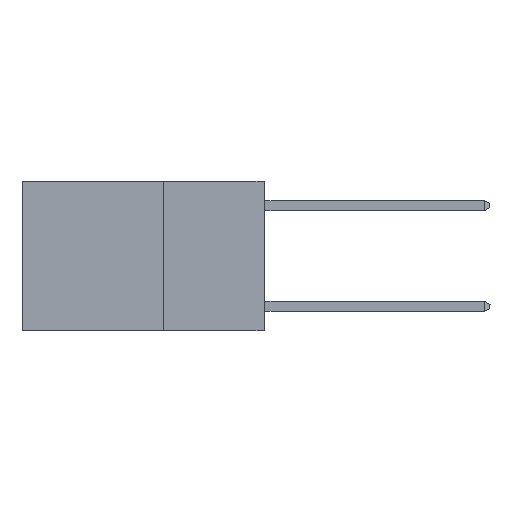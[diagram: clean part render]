
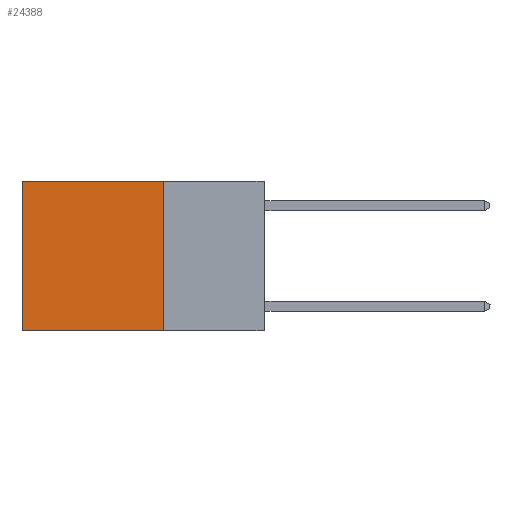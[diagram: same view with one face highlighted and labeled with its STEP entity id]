
A CAD part, left-side view. The second image highlights one B-rep face of the part: STEP entity #24388.
In plain terms, the highlighted planar face has unit normal (-1, 0, 0).
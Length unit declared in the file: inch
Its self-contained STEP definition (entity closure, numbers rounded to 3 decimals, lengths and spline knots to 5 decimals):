
#1171 = LINE ( 'NONE', #17954, #22110 ) ;
#3167 = VERTEX_POINT ( 'NONE', #11719 ) ;
#3984 = VERTEX_POINT ( 'NONE', #17899 ) ;
#4880 = VERTEX_POINT ( 'NONE', #18295 ) ;
#5075 = DIRECTION ( 'NONE',  ( 0., 1., 0. ) ) ;
#5185 = EDGE_CURVE ( 'NONE', #4880, #3984, #19962, .T. ) ;
#5824 = CARTESIAN_POINT ( 'NONE',  ( 0.2625, 0.25, 0. ) ) ;
#7811 = LINE ( 'NONE', #13350, #23177 ) ;
#8173 = PLANE ( 'NONE',  #19555 ) ;
#9255 = VECTOR ( 'NONE', #13308, 39.37008 ) ;
#10246 = CARTESIAN_POINT ( 'NONE',  ( 0.2625, 0.25, 0. ) ) ;
#11280 = CARTESIAN_POINT ( 'NONE',  ( 0.2625, 0.25, 0. ) ) ;
#11719 = CARTESIAN_POINT ( 'NONE',  ( 0.2625, 0.25, -0.37 ) ) ;
#11952 = ORIENTED_EDGE ( 'NONE', *, *, #17425, .T. ) ;
#12283 = CARTESIAN_POINT ( 'NONE',  ( 0.2625, 0.6, -0.37 ) ) ;
#12334 = DIRECTION ( 'NONE',  ( 0., 0., -1. ) ) ;
#13308 = DIRECTION ( 'NONE',  ( 0., 1., 0. ) ) ;
#13350 = CARTESIAN_POINT ( 'NONE',  ( 0.2625, 0.25, -0.37 ) ) ;
#14906 = EDGE_LOOP ( 'NONE', ( #11952, #21367, #20577, #20770 ) ) ;
#16794 = EDGE_CURVE ( 'NONE', #4880, #3167, #20734, .T. ) ;
#17425 = EDGE_CURVE ( 'NONE', #3984, #17508, #1171, .T. ) ;
#17508 = VERTEX_POINT ( 'NONE', #12283 ) ;
#17899 = CARTESIAN_POINT ( 'NONE',  ( 0.2625, 0.6, 0. ) ) ;
#17954 = CARTESIAN_POINT ( 'NONE',  ( 0.2625, 0.6, 0. ) ) ;
#18295 = CARTESIAN_POINT ( 'NONE',  ( 0.2625, 0.25, 0. ) ) ;
#19555 = AXIS2_PLACEMENT_3D ( 'NONE', #10246, #24158, #12334 ) ;
#19962 = LINE ( 'NONE', #11280, #9255 ) ;
#20018 = EDGE_CURVE ( 'NONE', #3167, #17508, #7811, .T. ) ;
#20117 = VECTOR ( 'NONE', #25884, 39.37008 ) ;
#20577 = ORIENTED_EDGE ( 'NONE', *, *, #16794, .F. ) ;
#20734 = LINE ( 'NONE', #5824, #20117 ) ;
#20770 = ORIENTED_EDGE ( 'NONE', *, *, #5185, .T. ) ;
#21367 = ORIENTED_EDGE ( 'NONE', *, *, #20018, .F. ) ;
#22110 = VECTOR ( 'NONE', #23857, 39.37008 ) ;
#23177 = VECTOR ( 'NONE', #5075, 39.37008 ) ;
#23857 = DIRECTION ( 'NONE',  ( 0., 0., -1. ) ) ;
#24158 = DIRECTION ( 'NONE',  ( 1., 0., 0. ) ) ;
#24388 = ADVANCED_FACE ( 'NONE', ( #25412 ), #8173, .F. ) ;
#25412 = FACE_OUTER_BOUND ( 'NONE', #14906, .T. ) ;
#25884 = DIRECTION ( 'NONE',  ( 0., 0., -1. ) ) ;
